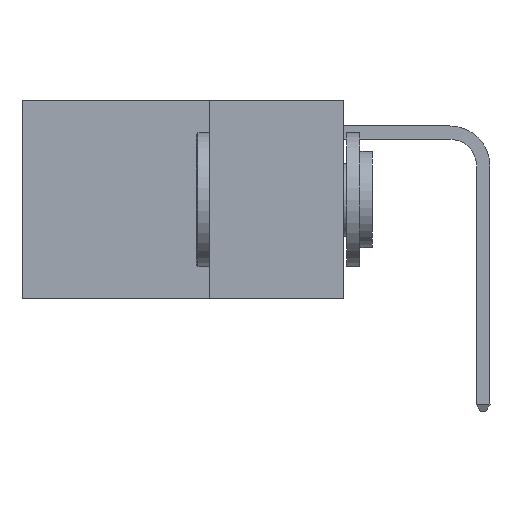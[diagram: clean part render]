
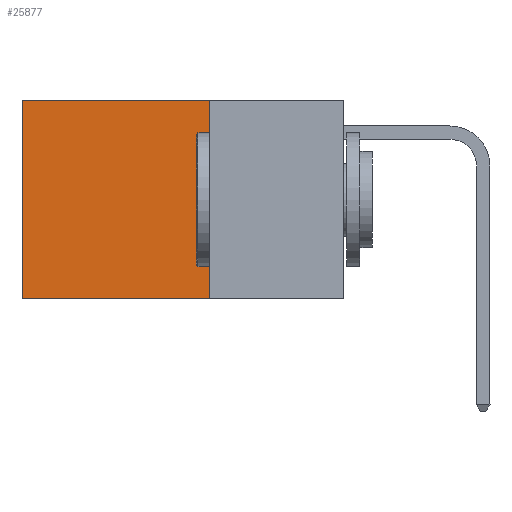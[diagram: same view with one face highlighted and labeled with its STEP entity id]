
A CAD part, left-side view. The second image highlights one B-rep face of the part: STEP entity #25877.
In plain terms, the highlighted planar face has unit normal (-1, 0, 0).
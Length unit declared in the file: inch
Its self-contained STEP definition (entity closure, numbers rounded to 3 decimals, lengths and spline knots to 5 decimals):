
#1612 = ORIENTED_EDGE ( 'NONE', *, *, #12881, .F. ) ;
#1951 = VECTOR ( 'NONE', #14484, 39.37008 ) ;
#2548 = EDGE_CURVE ( 'NONE', #23425, #8147, #23314, .T. ) ;
#2893 = ORIENTED_EDGE ( 'NONE', *, *, #14704, .T. ) ;
#3336 = DIRECTION ( 'NONE',  ( 0., 1., 0. ) ) ;
#3731 = PLANE ( 'NONE',  #16612 ) ;
#4375 = LINE ( 'NONE', #14480, #25694 ) ;
#4814 = EDGE_LOOP ( 'NONE', ( #6284, #14630, #1612, #2893 ) ) ;
#6284 = ORIENTED_EDGE ( 'NONE', *, *, #2548, .T. ) ;
#6788 = CARTESIAN_POINT ( 'NONE',  ( 0.2625, 0.6, -0.37 ) ) ;
#7479 = LINE ( 'NONE', #17710, #18130 ) ;
#8147 = VERTEX_POINT ( 'NONE', #6788 ) ;
#10144 = DIRECTION ( 'NONE',  ( 0., 0., -1. ) ) ;
#10884 = DIRECTION ( 'NONE',  ( 0., 1., 0. ) ) ;
#10900 = VERTEX_POINT ( 'NONE', #23196 ) ;
#11718 = EDGE_CURVE ( 'NONE', #18040, #8147, #4375, .T. ) ;
#11991 = LINE ( 'NONE', #16493, #1951 ) ;
#12881 = EDGE_CURVE ( 'NONE', #10900, #18040, #11991, .T. ) ;
#14213 = VECTOR ( 'NONE', #15295, 39.37008 ) ;
#14215 = CARTESIAN_POINT ( 'NONE',  ( 0.2625, 0.25, -0.37 ) ) ;
#14480 = CARTESIAN_POINT ( 'NONE',  ( 0.2625, 0.25, -0.37 ) ) ;
#14484 = DIRECTION ( 'NONE',  ( 0., 0., -1. ) ) ;
#14630 = ORIENTED_EDGE ( 'NONE', *, *, #11718, .F. ) ;
#14704 = EDGE_CURVE ( 'NONE', #10900, #23425, #7479, .T. ) ;
#15295 = DIRECTION ( 'NONE',  ( 0., 0., -1. ) ) ;
#16493 = CARTESIAN_POINT ( 'NONE',  ( 0.2625, 0.25, 0. ) ) ;
#16612 = AXIS2_PLACEMENT_3D ( 'NONE', #25910, #17842, #10144 ) ;
#17710 = CARTESIAN_POINT ( 'NONE',  ( 0.2625, 0.25, 0. ) ) ;
#17842 = DIRECTION ( 'NONE',  ( 1., 0., 0. ) ) ;
#18040 = VERTEX_POINT ( 'NONE', #14215 ) ;
#18130 = VECTOR ( 'NONE', #3336, 39.37008 ) ;
#21621 = CARTESIAN_POINT ( 'NONE',  ( 0.2625, 0.6, 0. ) ) ;
#22095 = FACE_OUTER_BOUND ( 'NONE', #4814, .T. ) ;
#23196 = CARTESIAN_POINT ( 'NONE',  ( 0.2625, 0.25, 0. ) ) ;
#23314 = LINE ( 'NONE', #25250, #14213 ) ;
#23425 = VERTEX_POINT ( 'NONE', #21621 ) ;
#25250 = CARTESIAN_POINT ( 'NONE',  ( 0.2625, 0.6, 0. ) ) ;
#25694 = VECTOR ( 'NONE', #10884, 39.37008 ) ;
#25877 = ADVANCED_FACE ( 'NONE', ( #22095 ), #3731, .F. ) ;
#25910 = CARTESIAN_POINT ( 'NONE',  ( 0.2625, 0.25, 0. ) ) ;
